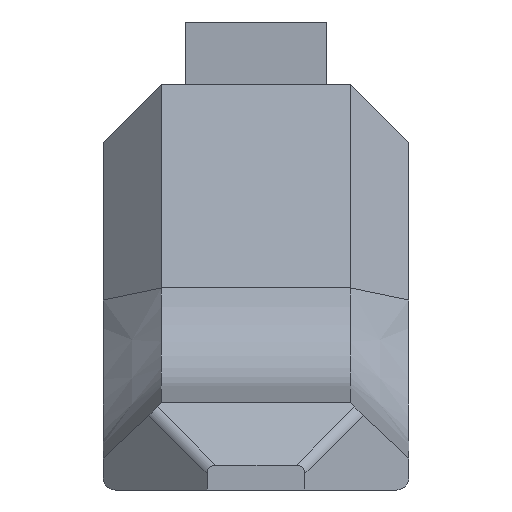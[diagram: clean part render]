
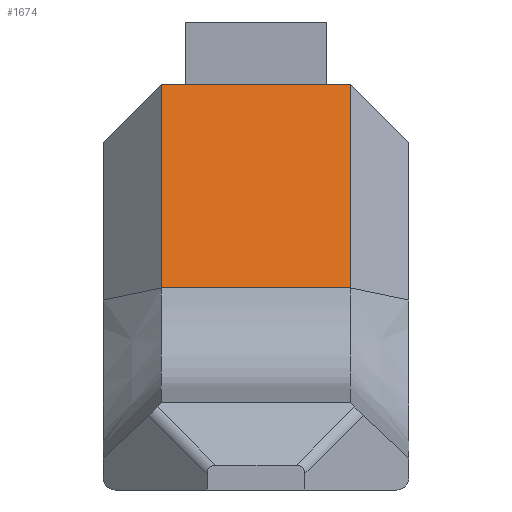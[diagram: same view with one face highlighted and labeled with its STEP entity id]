
A CAD part, front view. The second image highlights one B-rep face of the part: STEP entity #1674.
In plain terms, the highlighted planar face has unit normal (0, -0.978, 0.208).
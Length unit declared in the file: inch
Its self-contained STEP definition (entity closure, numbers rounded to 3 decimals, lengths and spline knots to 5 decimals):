
#45 = DIRECTION ( 'NONE',  ( 0., 0.208, 0.978 ) ) ;
#62 = CARTESIAN_POINT ( 'NONE',  ( 0.171, -2.48, 0.956 ) ) ;
#90 = CARTESIAN_POINT ( 'NONE',  ( 0., -2.48, 0.956 ) ) ;
#129 = EDGE_LOOP ( 'NONE', ( #1207, #1811, #467, #1940, #379, #749 ) ) ;
#196 = VECTOR ( 'NONE', #1273, 39.37008 ) ;
#293 = DIRECTION ( 'NONE',  ( 0., 0.208, 0.978 ) ) ;
#303 = DIRECTION ( 'NONE',  ( 1., 0., 0. ) ) ;
#314 = VERTEX_POINT ( 'NONE', #1939 ) ;
#331 = VERTEX_POINT ( 'NONE', #62 ) ;
#355 = FACE_OUTER_BOUND ( 'NONE', #129, .T. ) ;
#379 = ORIENTED_EDGE ( 'NONE', *, *, #1038, .F. ) ;
#447 = LINE ( 'NONE', #1117, #879 ) ;
#467 = ORIENTED_EDGE ( 'NONE', *, *, #1528, .T. ) ;
#596 = VECTOR ( 'NONE', #303, 39.37008 ) ;
#605 = DIRECTION ( 'NONE',  ( 0., -0.208, -0.978 ) ) ;
#640 = EDGE_CURVE ( 'NONE', #1500, #1631, #1289, .T. ) ;
#676 = EDGE_CURVE ( 'NONE', #2122, #331, #1794, .T. ) ;
#712 = PLANE ( 'NONE',  #1544 ) ;
#749 = ORIENTED_EDGE ( 'NONE', *, *, #676, .F. ) ;
#771 = CARTESIAN_POINT ( 'NONE',  ( -0.171, -2.48, 0.956 ) ) ;
#777 = CARTESIAN_POINT ( 'NONE',  ( -0.228, -2.48, 0.956 ) ) ;
#798 = CARTESIAN_POINT ( 'NONE',  ( -0.228, -2.58399, 0.46679 ) ) ;
#879 = VECTOR ( 'NONE', #293, 39.37008 ) ;
#883 = CARTESIAN_POINT ( 'NONE',  ( -0.368, -2.48, 0.956 ) ) ;
#1010 = VECTOR ( 'NONE', #2168, 39.37008 ) ;
#1038 = EDGE_CURVE ( 'NONE', #331, #1589, #1156, .T. ) ;
#1102 = LINE ( 'NONE', #1941, #596 ) ;
#1117 = CARTESIAN_POINT ( 'NONE',  ( 0.228, -2.48, 0.956 ) ) ;
#1156 = LINE ( 'NONE', #1671, #1010 ) ;
#1206 = VECTOR ( 'NONE', #605, 39.37008 ) ;
#1207 = ORIENTED_EDGE ( 'NONE', *, *, #2119, .F. ) ;
#1273 = DIRECTION ( 'NONE',  ( 1., 0., 0. ) ) ;
#1289 = LINE ( 'NONE', #1599, #1206 ) ;
#1453 = CARTESIAN_POINT ( 'NONE',  ( 0.368, -2.58399, 0.46679 ) ) ;
#1500 = VERTEX_POINT ( 'NONE', #777 ) ;
#1528 = EDGE_CURVE ( 'NONE', #1631, #314, #2083, .T. ) ;
#1544 = AXIS2_PLACEMENT_3D ( 'NONE', #883, #2040, #45 ) ;
#1589 = VERTEX_POINT ( 'NONE', #2028 ) ;
#1599 = CARTESIAN_POINT ( 'NONE',  ( -0.228, -2.48, 0.956 ) ) ;
#1631 = VERTEX_POINT ( 'NONE', #798 ) ;
#1671 = CARTESIAN_POINT ( 'NONE',  ( -0.368, -2.48, 0.956 ) ) ;
#1674 = ADVANCED_FACE ( 'NONE', ( #355 ), #712, .F. ) ;
#1794 = LINE ( 'NONE', #90, #196 ) ;
#1811 = ORIENTED_EDGE ( 'NONE', *, *, #640, .T. ) ;
#1939 = CARTESIAN_POINT ( 'NONE',  ( 0.228, -2.58399, 0.46679 ) ) ;
#1940 = ORIENTED_EDGE ( 'NONE', *, *, #2171, .T. ) ;
#1941 = CARTESIAN_POINT ( 'NONE',  ( -0.368, -2.48, 0.956 ) ) ;
#1967 = DIRECTION ( 'NONE',  ( 1., 0., 0. ) ) ;
#2028 = CARTESIAN_POINT ( 'NONE',  ( 0.228, -2.48, 0.956 ) ) ;
#2040 = DIRECTION ( 'NONE',  ( 0., 0.978, -0.208 ) ) ;
#2077 = VECTOR ( 'NONE', #1967, 39.37008 ) ;
#2083 = LINE ( 'NONE', #1453, #2077 ) ;
#2119 = EDGE_CURVE ( 'NONE', #1500, #2122, #1102, .T. ) ;
#2122 = VERTEX_POINT ( 'NONE', #771 ) ;
#2168 = DIRECTION ( 'NONE',  ( 1., 0., 0. ) ) ;
#2171 = EDGE_CURVE ( 'NONE', #314, #1589, #447, .T. ) ;
